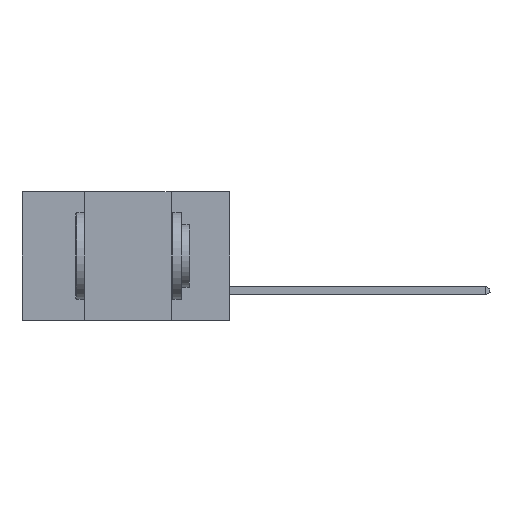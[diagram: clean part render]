
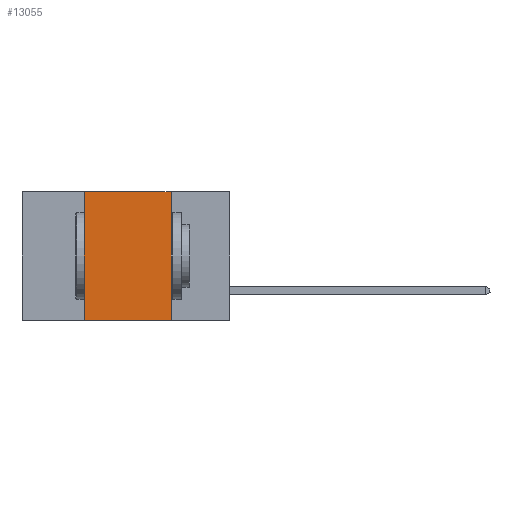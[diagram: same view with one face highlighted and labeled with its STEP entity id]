
A CAD part, left-side view. The second image highlights one B-rep face of the part: STEP entity #13055.
In plain terms, the highlighted planar face has unit normal (-1, 0, 0).
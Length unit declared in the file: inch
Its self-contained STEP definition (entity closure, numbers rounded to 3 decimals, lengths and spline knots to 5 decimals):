
#652 = ORIENTED_EDGE ( 'NONE', *, *, #916, .T. ) ;
#916 = EDGE_CURVE ( 'NONE', #12538, #5607, #1145, .T. ) ;
#1126 = EDGE_CURVE ( 'NONE', #5782, #5607, #10779, .T. ) ;
#1145 = LINE ( 'NONE', #15931, #9053 ) ;
#1544 = VERTEX_POINT ( 'NONE', #11336 ) ;
#1970 = LINE ( 'NONE', #4601, #6433 ) ;
#2425 = CARTESIAN_POINT ( 'NONE',  ( 0., 0.17, 0. ) ) ;
#2432 = DIRECTION ( 'NONE',  ( 0., -1., 0. ) ) ;
#3103 = DIRECTION ( 'NONE',  ( 1., 0., 0. ) ) ;
#4031 = LINE ( 'NONE', #7199, #9393 ) ;
#4601 = CARTESIAN_POINT ( 'NONE',  ( 0., 0.42, 0. ) ) ;
#4987 = ORIENTED_EDGE ( 'NONE', *, *, #10497, .F. ) ;
#5346 = EDGE_CURVE ( 'NONE', #12538, #1544, #1970, .T. ) ;
#5607 = VERTEX_POINT ( 'NONE', #7689 ) ;
#5782 = VERTEX_POINT ( 'NONE', #2425 ) ;
#6244 = DIRECTION ( 'NONE',  ( 0., -1., 0. ) ) ;
#6433 = VECTOR ( 'NONE', #7012, 39.37008 ) ;
#7012 = DIRECTION ( 'NONE',  ( 0., 0., 1. ) ) ;
#7016 = EDGE_LOOP ( 'NONE', ( #14987, #4987, #12799, #652 ) ) ;
#7199 = CARTESIAN_POINT ( 'NONE',  ( 0., 0.6, 0. ) ) ;
#7689 = CARTESIAN_POINT ( 'NONE',  ( 0., 0.17, -0.37 ) ) ;
#7702 = VECTOR ( 'NONE', #12250, 39.37008 ) ;
#7937 = PLANE ( 'NONE',  #14773 ) ;
#8548 = CARTESIAN_POINT ( 'NONE',  ( 0., 0.17, 0. ) ) ;
#9053 = VECTOR ( 'NONE', #2432, 39.37008 ) ;
#9393 = VECTOR ( 'NONE', #6244, 39.37008 ) ;
#10497 = EDGE_CURVE ( 'NONE', #1544, #5782, #4031, .T. ) ;
#10779 = LINE ( 'NONE', #8548, #7702 ) ;
#11336 = CARTESIAN_POINT ( 'NONE',  ( 0., 0.42, 0. ) ) ;
#12250 = DIRECTION ( 'NONE',  ( 0., 0., -1. ) ) ;
#12538 = VERTEX_POINT ( 'NONE', #12543 ) ;
#12543 = CARTESIAN_POINT ( 'NONE',  ( 0., 0.42, -0.37 ) ) ;
#12799 = ORIENTED_EDGE ( 'NONE', *, *, #5346, .F. ) ;
#13055 = ADVANCED_FACE ( 'NONE', ( #13800 ), #7937, .F. ) ;
#13800 = FACE_OUTER_BOUND ( 'NONE', #7016, .T. ) ;
#14225 = CARTESIAN_POINT ( 'NONE',  ( 0., 0.6, 0. ) ) ;
#14773 = AXIS2_PLACEMENT_3D ( 'NONE', #14225, #3103, #15280 ) ;
#14987 = ORIENTED_EDGE ( 'NONE', *, *, #1126, .F. ) ;
#15280 = DIRECTION ( 'NONE',  ( 0., 0., -1. ) ) ;
#15931 = CARTESIAN_POINT ( 'NONE',  ( 0., 0.6, -0.37 ) ) ;
